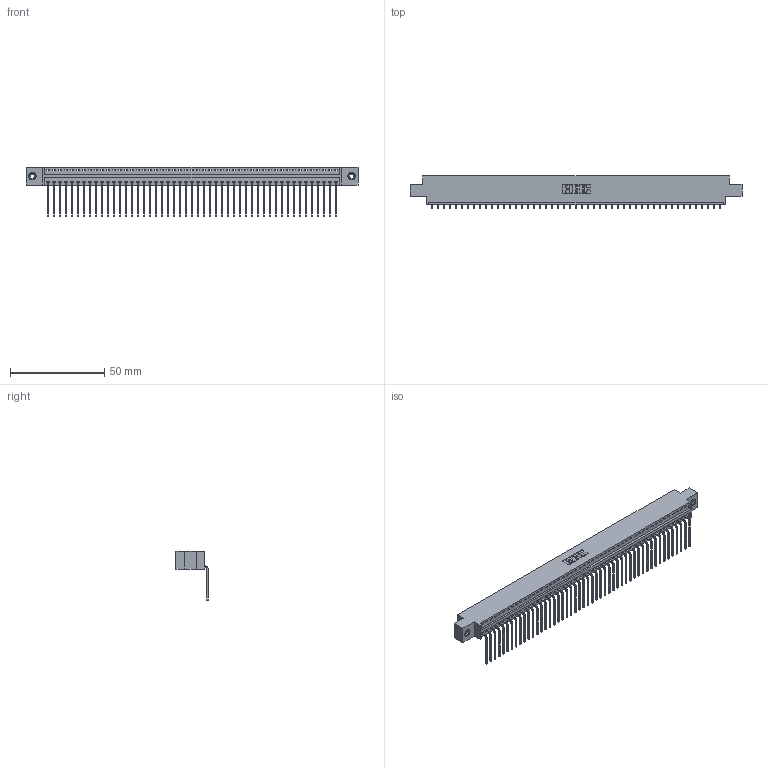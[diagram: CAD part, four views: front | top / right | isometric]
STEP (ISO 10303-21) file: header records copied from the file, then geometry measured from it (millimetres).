
FILE_DESCRIPTION (( 'STEP AP203' ), '1' );
FILE_NAME ('346-049-559-608.STEP', '2022-05-10T02:22:03', ( '' ), ( '' ), 'SwSTEP 2.0', 'SolidWorks 2020', '' );
FILE_SCHEMA (( 'CONFIG_CONTROL_DESIGN' ));
Length unit declared in the file: inch
Products named in the file (4): 345-292-001_558 559 Tail - 1; 346 Part_0.170 Offset - 0.156 Dia-TI; 346-049-559-608; 345-250-001_345-250-003-102
Assembly tree (52 placements, depth 2):
  346-049-559-608
    346 Part_0.170 Offset - 0.156 Dia-TI
    345-292-001_558 559 Tail - 1  x49
    345-250-001_345-250-003-102  x2
Bounding box: 176.15 x 17.08 x 26.16 mm (x, y, z)
Volume: 16911.7 mm3; surface area: 22369.1 mm2
Topology: 52 solids, 52 shells, 3126 faces, 9395 edges, 6190 vertices
Faces by surface type: plane 2170, cylinder 940, cone 12, torus 4
Entity records: 30870 total; most frequent: CARTESIAN_POINT 5274, ORIENTED_EDGE 5250, DIRECTION 4669, EDGE_CURVE 2625, VECTOR 2277, LINE 2277, VERTEX_POINT 1744, AXIS2_PLACEMENT_3D 1196
